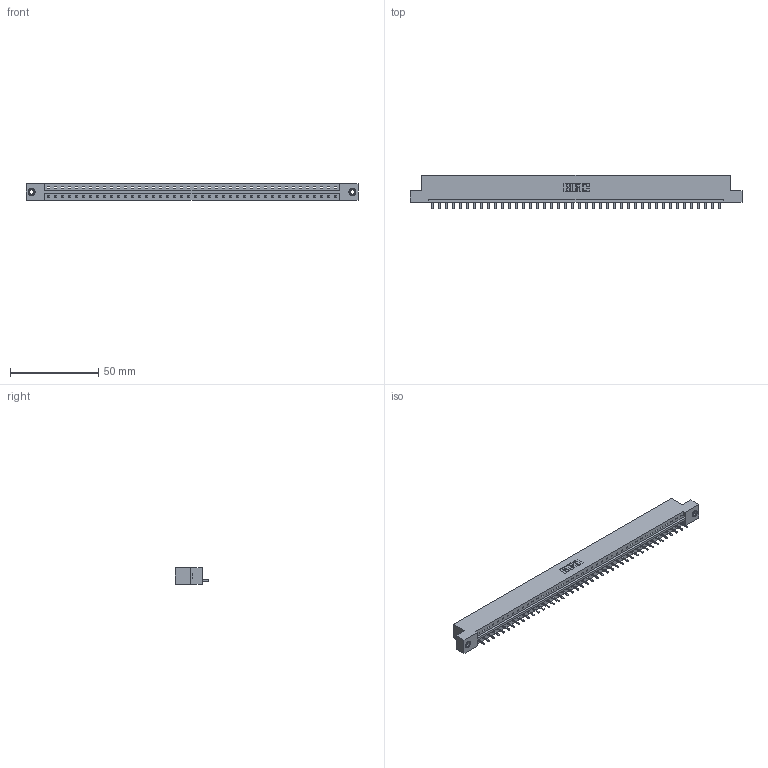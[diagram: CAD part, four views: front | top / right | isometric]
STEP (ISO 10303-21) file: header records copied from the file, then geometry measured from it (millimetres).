
FILE_DESCRIPTION (( 'STEP AP203' ), '1' );
FILE_NAME ('833-042-521-107.STEP', '2020-06-03T20:25:20', ( '' ), ( '' ), 'SwSTEP 2.0', 'SolidWorks 2020', '' );
FILE_SCHEMA (( 'CONFIG_CONTROL_DESIGN' ));
Length unit declared in the file: inch
Products named in the file (4): 833 Part_Flush - .156 Dia - TI; 345-292-001_345-293-121; 833-042-521-107; 345-250-001_345-250-005-103
Assembly tree (45 placements, depth 2):
  833-042-521-107
    833 Part_Flush - .156 Dia - TI
    345-292-001_345-293-121  x42
    345-250-001_345-250-005-103  x2
Bounding box: 187.96 x 19.06 x 9.4 mm (x, y, z)
Volume: 18781.1 mm3; surface area: 19862.8 mm2
Topology: 45 solids, 45 shells, 2610 faces, 7839 edges, 5162 vertices
Faces by surface type: plane 1866, cylinder 728, cone 12, torus 4
Entity records: 26880 total; most frequent: CARTESIAN_POINT 4619, ORIENTED_EDGE 4590, DIRECTION 3929, EDGE_CURVE 2295, VECTOR 2147, LINE 2147, VERTEX_POINT 1524, AXIS2_PLACEMENT_3D 891
